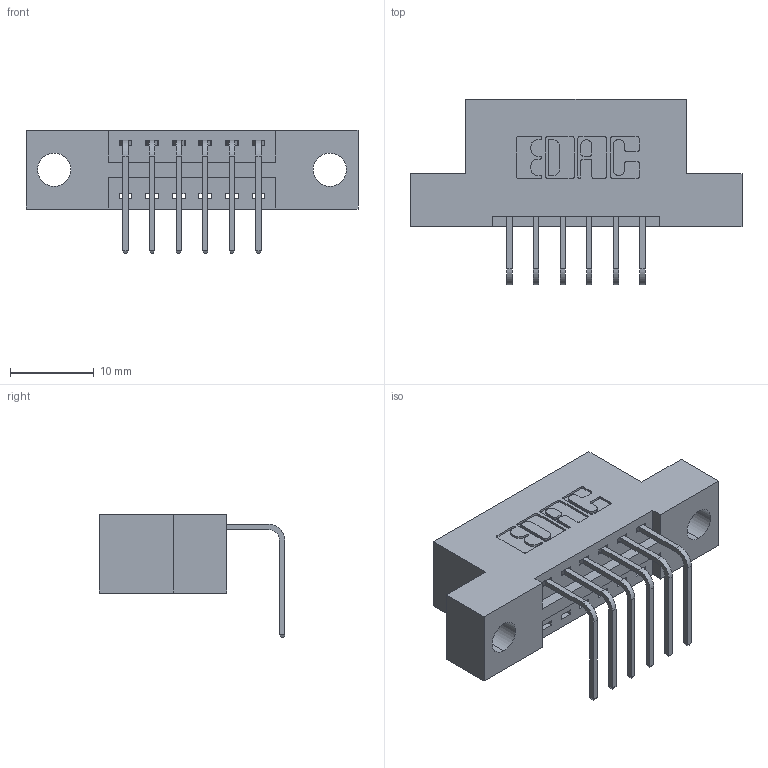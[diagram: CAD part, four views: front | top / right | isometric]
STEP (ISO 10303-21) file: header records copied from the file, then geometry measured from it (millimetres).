
FILE_DESCRIPTION (( 'STEP AP203' ), '1' );
FILE_NAME ('396-006-558-104.STEP', '2022-05-17T05:43:24', ( '' ), ( '' ), 'SwSTEP 2.0', 'SolidWorks 2020', '' );
FILE_SCHEMA (( 'CONFIG_CONTROL_DESIGN' ));
Length unit declared in the file: inch
Products named in the file (3): 396-006-558-104; 346 Part_Flush Mounting Lugs - 0.156 Dia-TH; 345-292-001_558 Tail - 2
Assembly tree (7 placements, depth 2):
  396-006-558-104
    346 Part_Flush Mounting Lugs - 0.156 Dia-TH
    345-292-001_558 Tail - 2  x6
Bounding box: 39.62 x 22.16 x 14.73 mm (x, y, z)
Volume: 3458.9 mm3; surface area: 3891.2 mm2
Topology: 7 solids, 7 shells, 496 faces, 1457 edges, 962 vertices
Faces by surface type: plane 342, cylinder 154
Entity records: 9073 total; most frequent: CARTESIAN_POINT 1576, ORIENTED_EDGE 1514, DIRECTION 1433, EDGE_CURVE 757, LINE 601, VECTOR 601, VERTEX_POINT 502, AXIS2_PLACEMENT_3D 416
